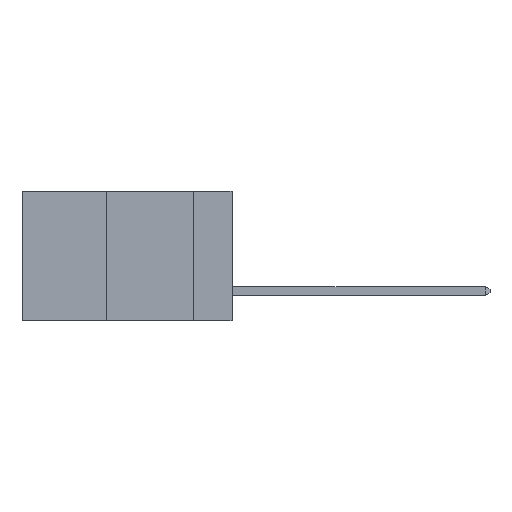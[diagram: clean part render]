
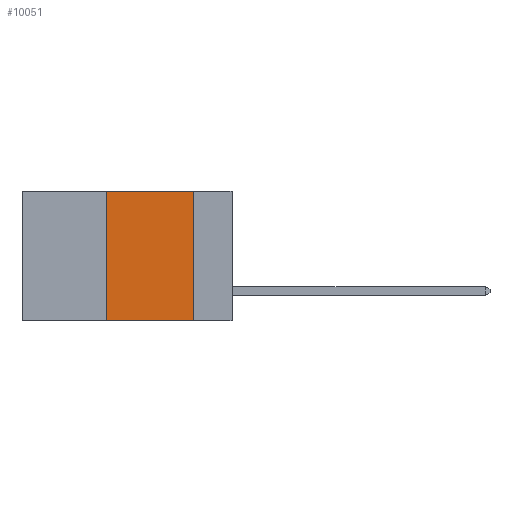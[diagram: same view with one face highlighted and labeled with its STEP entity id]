
A CAD part, left-side view. The second image highlights one B-rep face of the part: STEP entity #10051.
In plain terms, the highlighted planar face has unit normal (-1, 0, 0).
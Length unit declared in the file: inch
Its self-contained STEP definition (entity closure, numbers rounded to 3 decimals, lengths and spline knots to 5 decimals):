
#32 = CARTESIAN_POINT ( 'NONE',  ( 0., 0.36, 0. ) ) ;
#663 = LINE ( 'NONE', #7118, #4209 ) ;
#2296 = DIRECTION ( 'NONE',  ( 0., 0., -1. ) ) ;
#2944 = VERTEX_POINT ( 'NONE', #32 ) ;
#2988 = LINE ( 'NONE', #7503, #7885 ) ;
#3293 = FACE_OUTER_BOUND ( 'NONE', #7871, .T. ) ;
#3303 = VERTEX_POINT ( 'NONE', #10775 ) ;
#4209 = VECTOR ( 'NONE', #5516, 39.37008 ) ;
#4731 = EDGE_CURVE ( 'NONE', #5717, #2944, #663, .T. ) ;
#5136 = LINE ( 'NONE', #5465, #5752 ) ;
#5403 = DIRECTION ( 'NONE',  ( 0., 0., -1. ) ) ;
#5465 = CARTESIAN_POINT ( 'NONE',  ( 0., 0.6, -0.37 ) ) ;
#5516 = DIRECTION ( 'NONE',  ( 0., 0., 1. ) ) ;
#5717 = VERTEX_POINT ( 'NONE', #6643 ) ;
#5752 = VECTOR ( 'NONE', #7828, 39.37008 ) ;
#6048 = EDGE_CURVE ( 'NONE', #5717, #3303, #5136, .T. ) ;
#6261 = VECTOR ( 'NONE', #5403, 39.37008 ) ;
#6292 = PLANE ( 'NONE',  #10037 ) ;
#6643 = CARTESIAN_POINT ( 'NONE',  ( 0., 0.36, -0.37 ) ) ;
#6898 = ORIENTED_EDGE ( 'NONE', *, *, #9146, .F. ) ;
#7118 = CARTESIAN_POINT ( 'NONE',  ( 0., 0.36, 0. ) ) ;
#7189 = ORIENTED_EDGE ( 'NONE', *, *, #6048, .T. ) ;
#7238 = CARTESIAN_POINT ( 'NONE',  ( 0., 0.6, 0. ) ) ;
#7503 = CARTESIAN_POINT ( 'NONE',  ( 0., 0.6, 0. ) ) ;
#7828 = DIRECTION ( 'NONE',  ( 0., -1., 0. ) ) ;
#7871 = EDGE_LOOP ( 'NONE', ( #6898, #11630, #9350, #7189 ) ) ;
#7885 = VECTOR ( 'NONE', #8422, 39.37008 ) ;
#8169 = DIRECTION ( 'NONE',  ( 1., 0., 0. ) ) ;
#8422 = DIRECTION ( 'NONE',  ( 0., -1., 0. ) ) ;
#9146 = EDGE_CURVE ( 'NONE', #10263, #3303, #10855, .T. ) ;
#9350 = ORIENTED_EDGE ( 'NONE', *, *, #4731, .F. ) ;
#10037 = AXIS2_PLACEMENT_3D ( 'NONE', #7238, #8169, #2296 ) ;
#10051 = ADVANCED_FACE ( 'NONE', ( #3293 ), #6292, .F. ) ;
#10263 = VERTEX_POINT ( 'NONE', #11928 ) ;
#10775 = CARTESIAN_POINT ( 'NONE',  ( 0., 0.11, -0.37 ) ) ;
#10855 = LINE ( 'NONE', #11705, #6261 ) ;
#11283 = EDGE_CURVE ( 'NONE', #2944, #10263, #2988, .T. ) ;
#11630 = ORIENTED_EDGE ( 'NONE', *, *, #11283, .F. ) ;
#11705 = CARTESIAN_POINT ( 'NONE',  ( 0., 0.11, 0. ) ) ;
#11928 = CARTESIAN_POINT ( 'NONE',  ( 0., 0.11, 0. ) ) ;
